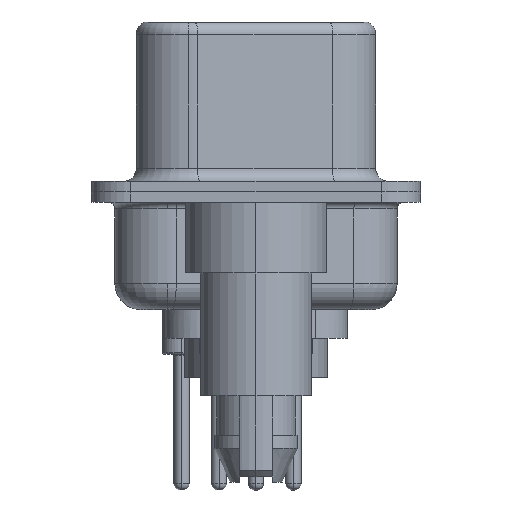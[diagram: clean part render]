
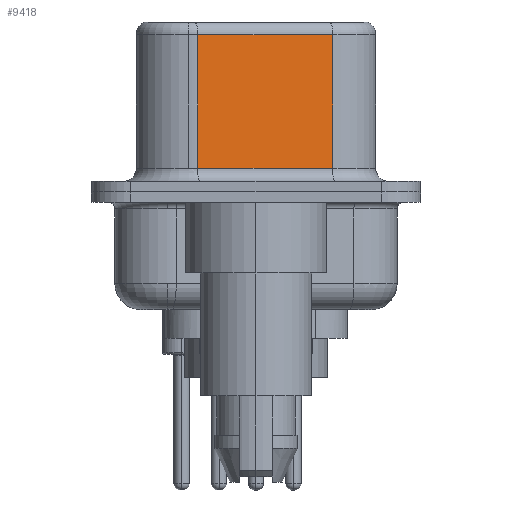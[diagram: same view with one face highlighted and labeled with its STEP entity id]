
A CAD part, left-side view. The second image highlights one B-rep face of the part: STEP entity #9418.
In plain terms, the highlighted planar face has unit normal (-0.985, -0.174, 0).
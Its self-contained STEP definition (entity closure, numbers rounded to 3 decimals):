
#1040 = LINE ( 'NONE', #1638, #1285 ) ;
#1285 = VECTOR ( 'NONE', #4944, 1000. ) ;
#1638 = CARTESIAN_POINT ( 'NONE',  ( 4.585, -2.927, 6.02 ) ) ;
#1810 = EDGE_CURVE ( 'NONE', #20787, #11808, #11019, .T. ) ;
#2245 = CARTESIAN_POINT ( 'NONE',  ( 4.585, -2.927, 0.9 ) ) ;
#2797 = ORIENTED_EDGE ( 'NONE', *, *, #12533, .T. ) ;
#3444 = CARTESIAN_POINT ( 'NONE',  ( 4.585, -2.927, 6.52 ) ) ;
#3589 = ORIENTED_EDGE ( 'NONE', *, *, #18533, .T. ) ;
#3666 = DIRECTION ( 'NONE',  ( 0.174, -0.985, 0. ) ) ;
#4809 = LINE ( 'NONE', #3444, #6351 ) ;
#4944 = DIRECTION ( 'NONE',  ( -0.174, 0.985, 0. ) ) ;
#6351 = VECTOR ( 'NONE', #10049, 1000. ) ;
#6533 = PLANE ( 'NONE',  #14870 ) ;
#7513 = EDGE_LOOP ( 'NONE', ( #18792, #3589, #19007, #2797 ) ) ;
#7909 = EDGE_CURVE ( 'NONE', #19293, #20997, #4809, .T. ) ;
#8404 = CARTESIAN_POINT ( 'NONE',  ( 3.675, 2.233, 6.02 ) ) ;
#8755 = VECTOR ( 'NONE', #20949, 1000. ) ;
#9418 = ADVANCED_FACE ( 'NONE', ( #18501 ), #6533, .F. ) ;
#10049 = DIRECTION ( 'NONE',  ( 0., 0., -1. ) ) ;
#10888 = CARTESIAN_POINT ( 'NONE',  ( 3.675, 2.233, 6.52 ) ) ;
#11019 = LINE ( 'NONE', #10888, #8755 ) ;
#11808 = VERTEX_POINT ( 'NONE', #19665 ) ;
#12533 = EDGE_CURVE ( 'NONE', #11808, #20997, #20485, .T. ) ;
#12856 = CARTESIAN_POINT ( 'NONE',  ( 4.585, -2.927, 6.02 ) ) ;
#14870 = AXIS2_PLACEMENT_3D ( 'NONE', #18034, #21359, #16437 ) ;
#15477 = CARTESIAN_POINT ( 'NONE',  ( 4.585, -2.927, 0.9 ) ) ;
#16437 = DIRECTION ( 'NONE',  ( -0.174, 0.985, 0. ) ) ;
#16853 = VECTOR ( 'NONE', #3666, 1000. ) ;
#18034 = CARTESIAN_POINT ( 'NONE',  ( 4.585, -2.927, 6.52 ) ) ;
#18501 = FACE_OUTER_BOUND ( 'NONE', #7513, .T. ) ;
#18533 = EDGE_CURVE ( 'NONE', #19293, #20787, #1040, .T. ) ;
#18792 = ORIENTED_EDGE ( 'NONE', *, *, #7909, .F. ) ;
#19007 = ORIENTED_EDGE ( 'NONE', *, *, #1810, .T. ) ;
#19293 = VERTEX_POINT ( 'NONE', #12856 ) ;
#19665 = CARTESIAN_POINT ( 'NONE',  ( 3.675, 2.233, 0.9 ) ) ;
#20485 = LINE ( 'NONE', #15477, #16853 ) ;
#20787 = VERTEX_POINT ( 'NONE', #8404 ) ;
#20949 = DIRECTION ( 'NONE',  ( 0., 0., -1. ) ) ;
#20997 = VERTEX_POINT ( 'NONE', #2245 ) ;
#21359 = DIRECTION ( 'NONE',  ( 0.985, 0.174, 0. ) ) ;
